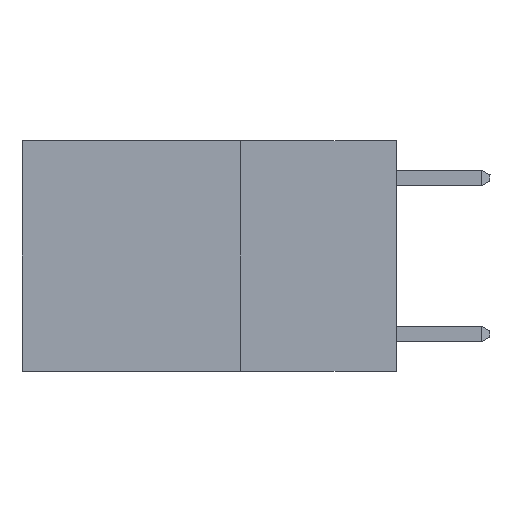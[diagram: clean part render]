
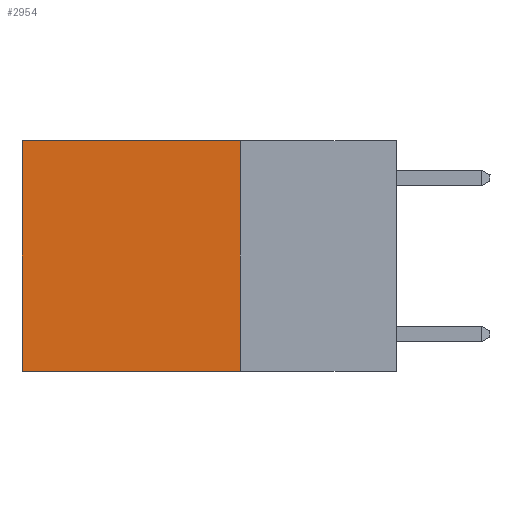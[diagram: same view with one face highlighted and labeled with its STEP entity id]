
A CAD part, left-side view. The second image highlights one B-rep face of the part: STEP entity #2954.
In plain terms, the highlighted planar face has unit normal (-1, 0, 0).
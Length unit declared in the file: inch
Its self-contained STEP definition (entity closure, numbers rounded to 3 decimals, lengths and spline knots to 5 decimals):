
#6 = VECTOR ( 'NONE', #10058, 39.37008 ) ;
#403 = VERTEX_POINT ( 'NONE', #16558 ) ;
#815 = VECTOR ( 'NONE', #6601, 39.37008 ) ;
#2005 = PLANE ( 'NONE',  #9388 ) ;
#2954 = ADVANCED_FACE ( 'NONE', ( #9519 ), #2005, .F. ) ;
#4036 = DIRECTION ( 'NONE',  ( 0., 0., -1. ) ) ;
#4630 = VERTEX_POINT ( 'NONE', #16777 ) ;
#4715 = DIRECTION ( 'NONE',  ( 0., 0., -1. ) ) ;
#4990 = EDGE_CURVE ( 'NONE', #17287, #12820, #10957, .T. ) ;
#5149 = LINE ( 'NONE', #24317, #25342 ) ;
#6106 = ORIENTED_EDGE ( 'NONE', *, *, #7492, .T. ) ;
#6601 = DIRECTION ( 'NONE',  ( 0., 0., -1. ) ) ;
#7391 = ORIENTED_EDGE ( 'NONE', *, *, #24432, .F. ) ;
#7492 = EDGE_CURVE ( 'NONE', #12820, #403, #21326, .T. ) ;
#8271 = EDGE_LOOP ( 'NONE', ( #6106, #7391, #18996, #25512 ) ) ;
#9388 = AXIS2_PLACEMENT_3D ( 'NONE', #21723, #15954, #4036 ) ;
#9519 = FACE_OUTER_BOUND ( 'NONE', #8271, .T. ) ;
#9831 = DIRECTION ( 'NONE',  ( 0., 1., 0. ) ) ;
#10058 = DIRECTION ( 'NONE',  ( 0., 1., 0. ) ) ;
#10957 = LINE ( 'NONE', #23491, #15627 ) ;
#12820 = VERTEX_POINT ( 'NONE', #14549 ) ;
#14056 = EDGE_CURVE ( 'NONE', #17287, #4630, #5149, .T. ) ;
#14167 = LINE ( 'NONE', #19909, #6 ) ;
#14549 = CARTESIAN_POINT ( 'NONE',  ( 0.2625, 0.6, 0. ) ) ;
#15627 = VECTOR ( 'NONE', #9831, 39.37008 ) ;
#15954 = DIRECTION ( 'NONE',  ( 1., 0., 0. ) ) ;
#16558 = CARTESIAN_POINT ( 'NONE',  ( 0.2625, 0.6, -0.37 ) ) ;
#16777 = CARTESIAN_POINT ( 'NONE',  ( 0.2625, 0.25, -0.37 ) ) ;
#17287 = VERTEX_POINT ( 'NONE', #23275 ) ;
#18996 = ORIENTED_EDGE ( 'NONE', *, *, #14056, .F. ) ;
#19909 = CARTESIAN_POINT ( 'NONE',  ( 0.2625, 0.25, -0.37 ) ) ;
#21326 = LINE ( 'NONE', #22353, #815 ) ;
#21723 = CARTESIAN_POINT ( 'NONE',  ( 0.2625, 0.25, 0. ) ) ;
#22353 = CARTESIAN_POINT ( 'NONE',  ( 0.2625, 0.6, 0. ) ) ;
#23275 = CARTESIAN_POINT ( 'NONE',  ( 0.2625, 0.25, 0. ) ) ;
#23491 = CARTESIAN_POINT ( 'NONE',  ( 0.2625, 0.25, 0. ) ) ;
#24317 = CARTESIAN_POINT ( 'NONE',  ( 0.2625, 0.25, 0. ) ) ;
#24432 = EDGE_CURVE ( 'NONE', #4630, #403, #14167, .T. ) ;
#25342 = VECTOR ( 'NONE', #4715, 39.37008 ) ;
#25512 = ORIENTED_EDGE ( 'NONE', *, *, #4990, .T. ) ;
